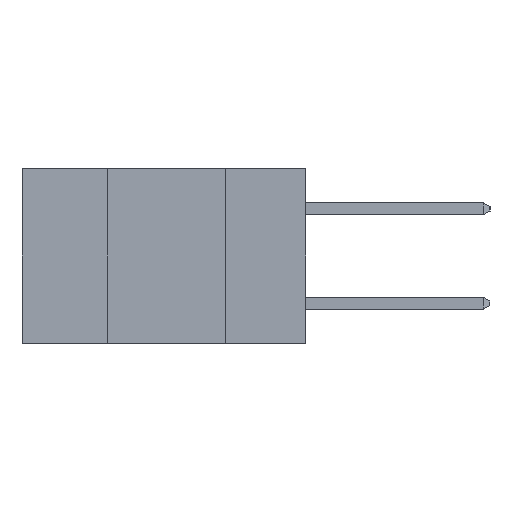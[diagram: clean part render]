
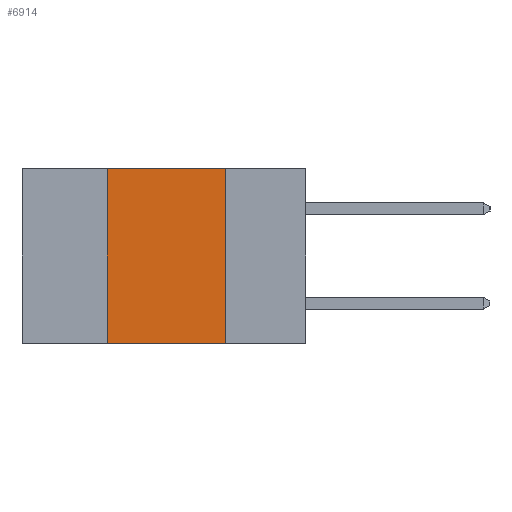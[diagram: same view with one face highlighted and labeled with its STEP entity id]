
A CAD part, left-side view. The second image highlights one B-rep face of the part: STEP entity #6914.
In plain terms, the highlighted planar face has unit normal (-1, 0, 0).
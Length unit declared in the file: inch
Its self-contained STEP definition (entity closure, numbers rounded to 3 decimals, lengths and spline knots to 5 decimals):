
#265 = CARTESIAN_POINT ( 'NONE',  ( 0., 0.17, 0. ) ) ;
#474 = CARTESIAN_POINT ( 'NONE',  ( 0., 0.42, -0.37 ) ) ;
#749 = FACE_OUTER_BOUND ( 'NONE', #9802, .T. ) ;
#1334 = ORIENTED_EDGE ( 'NONE', *, *, #9076, .F. ) ;
#1397 = ORIENTED_EDGE ( 'NONE', *, *, #3345, .F. ) ;
#1517 = EDGE_CURVE ( 'NONE', #10355, #3558, #5302, .T. ) ;
#3069 = VECTOR ( 'NONE', #3138, 39.37008 ) ;
#3138 = DIRECTION ( 'NONE',  ( 0., -1., 0. ) ) ;
#3345 = EDGE_CURVE ( 'NONE', #3542, #6533, #5376, .T. ) ;
#3542 = VERTEX_POINT ( 'NONE', #8637 ) ;
#3558 = VERTEX_POINT ( 'NONE', #9827 ) ;
#3601 = CARTESIAN_POINT ( 'NONE',  ( 0., 0.6, 0. ) ) ;
#4444 = DIRECTION ( 'NONE',  ( 1., 0., 0. ) ) ;
#4683 = EDGE_CURVE ( 'NONE', #10355, #3542, #7696, .T. ) ;
#4936 = CARTESIAN_POINT ( 'NONE',  ( 0., 0.6, 0. ) ) ;
#4949 = AXIS2_PLACEMENT_3D ( 'NONE', #3601, #4444, #5489 ) ;
#5061 = VECTOR ( 'NONE', #8674, 39.37008 ) ;
#5302 = LINE ( 'NONE', #10299, #3069 ) ;
#5376 = LINE ( 'NONE', #4936, #7468 ) ;
#5489 = DIRECTION ( 'NONE',  ( 0., 0., -1. ) ) ;
#6085 = CARTESIAN_POINT ( 'NONE',  ( 0., 0.42, 0. ) ) ;
#6533 = VERTEX_POINT ( 'NONE', #265 ) ;
#6914 = ADVANCED_FACE ( 'NONE', ( #749 ), #10283, .F. ) ;
#7468 = VECTOR ( 'NONE', #8881, 39.37008 ) ;
#7620 = ORIENTED_EDGE ( 'NONE', *, *, #4683, .F. ) ;
#7665 = VECTOR ( 'NONE', #8652, 39.37008 ) ;
#7696 = LINE ( 'NONE', #6085, #5061 ) ;
#8637 = CARTESIAN_POINT ( 'NONE',  ( 0., 0.42, 0. ) ) ;
#8652 = DIRECTION ( 'NONE',  ( 0., 0., -1. ) ) ;
#8674 = DIRECTION ( 'NONE',  ( 0., 0., 1. ) ) ;
#8881 = DIRECTION ( 'NONE',  ( 0., -1., 0. ) ) ;
#9076 = EDGE_CURVE ( 'NONE', #6533, #3558, #9776, .T. ) ;
#9333 = ORIENTED_EDGE ( 'NONE', *, *, #1517, .T. ) ;
#9400 = CARTESIAN_POINT ( 'NONE',  ( 0., 0.17, 0. ) ) ;
#9776 = LINE ( 'NONE', #9400, #7665 ) ;
#9802 = EDGE_LOOP ( 'NONE', ( #1334, #1397, #7620, #9333 ) ) ;
#9827 = CARTESIAN_POINT ( 'NONE',  ( 0., 0.17, -0.37 ) ) ;
#10283 = PLANE ( 'NONE',  #4949 ) ;
#10299 = CARTESIAN_POINT ( 'NONE',  ( 0., 0.6, -0.37 ) ) ;
#10355 = VERTEX_POINT ( 'NONE', #474 ) ;
